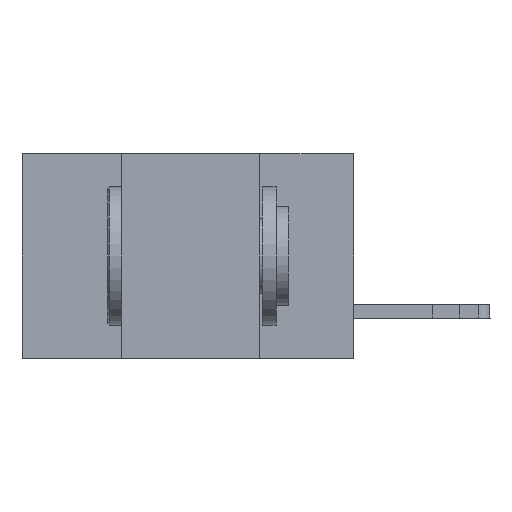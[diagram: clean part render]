
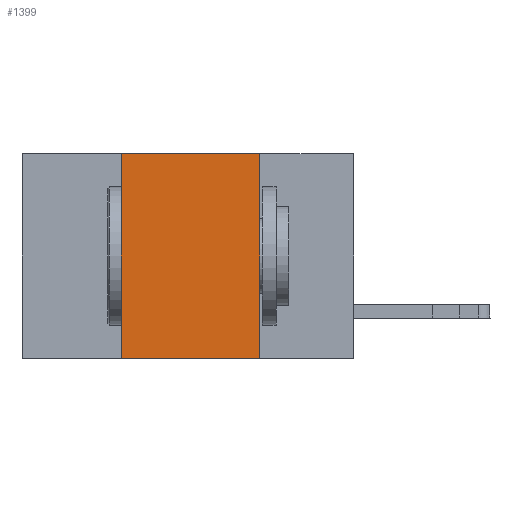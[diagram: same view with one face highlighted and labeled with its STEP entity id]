
A CAD part, left-side view. The second image highlights one B-rep face of the part: STEP entity #1399.
In plain terms, the highlighted planar face has unit normal (-1, 0, 0).
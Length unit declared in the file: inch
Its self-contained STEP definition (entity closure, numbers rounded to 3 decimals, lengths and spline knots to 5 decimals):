
#641 = CARTESIAN_POINT ( 'NONE',  ( 0., 0.6, -0.37 ) ) ;
#858 = DIRECTION ( 'NONE',  ( 0., 0., 1. ) ) ;
#898 = DIRECTION ( 'NONE',  ( 0., -1., 0. ) ) ;
#1149 = AXIS2_PLACEMENT_3D ( 'NONE', #9027, #26826, #27082 ) ;
#1399 = ADVANCED_FACE ( 'NONE', ( #32312 ), #5887, .F. ) ;
#2124 = CARTESIAN_POINT ( 'NONE',  ( 0., 0.17, -0.37 ) ) ;
#3945 = ORIENTED_EDGE ( 'NONE', *, *, #27786, .F. ) ;
#4707 = CARTESIAN_POINT ( 'NONE',  ( 0., 0.6, 0. ) ) ;
#5061 = ORIENTED_EDGE ( 'NONE', *, *, #26195, .F. ) ;
#5376 = CARTESIAN_POINT ( 'NONE',  ( 0., 0.42, -0.37 ) ) ;
#5887 = PLANE ( 'NONE',  #1149 ) ;
#9027 = CARTESIAN_POINT ( 'NONE',  ( 0., 0.6, 0. ) ) ;
#9453 = LINE ( 'NONE', #641, #12631 ) ;
#10197 = DIRECTION ( 'NONE',  ( 0., -1., 0. ) ) ;
#10820 = VECTOR ( 'NONE', #858, 39.37008 ) ;
#12631 = VECTOR ( 'NONE', #898, 39.37008 ) ;
#12920 = VECTOR ( 'NONE', #15961, 39.37008 ) ;
#15961 = DIRECTION ( 'NONE',  ( 0., 0., -1. ) ) ;
#18323 = EDGE_CURVE ( 'NONE', #25754, #30664, #9453, .T. ) ;
#18326 = VECTOR ( 'NONE', #10197, 39.37008 ) ;
#18412 = VERTEX_POINT ( 'NONE', #37747 ) ;
#18489 = LINE ( 'NONE', #35793, #10820 ) ;
#19053 = EDGE_CURVE ( 'NONE', #25754, #18412, #18489, .T. ) ;
#21118 = LINE ( 'NONE', #4707, #18326 ) ;
#25338 = EDGE_LOOP ( 'NONE', ( #5061, #3945, #36232, #26390 ) ) ;
#25754 = VERTEX_POINT ( 'NONE', #5376 ) ;
#26195 = EDGE_CURVE ( 'NONE', #26576, #30664, #33552, .T. ) ;
#26390 = ORIENTED_EDGE ( 'NONE', *, *, #18323, .T. ) ;
#26576 = VERTEX_POINT ( 'NONE', #35657 ) ;
#26826 = DIRECTION ( 'NONE',  ( 1., 0., 0. ) ) ;
#27082 = DIRECTION ( 'NONE',  ( 0., 0., -1. ) ) ;
#27786 = EDGE_CURVE ( 'NONE', #18412, #26576, #21118, .T. ) ;
#30664 = VERTEX_POINT ( 'NONE', #2124 ) ;
#32312 = FACE_OUTER_BOUND ( 'NONE', #25338, .T. ) ;
#33530 = CARTESIAN_POINT ( 'NONE',  ( 0., 0.17, 0. ) ) ;
#33552 = LINE ( 'NONE', #33530, #12920 ) ;
#35657 = CARTESIAN_POINT ( 'NONE',  ( 0., 0.17, 0. ) ) ;
#35793 = CARTESIAN_POINT ( 'NONE',  ( 0., 0.42, 0. ) ) ;
#36232 = ORIENTED_EDGE ( 'NONE', *, *, #19053, .F. ) ;
#37747 = CARTESIAN_POINT ( 'NONE',  ( 0., 0.42, 0. ) ) ;
